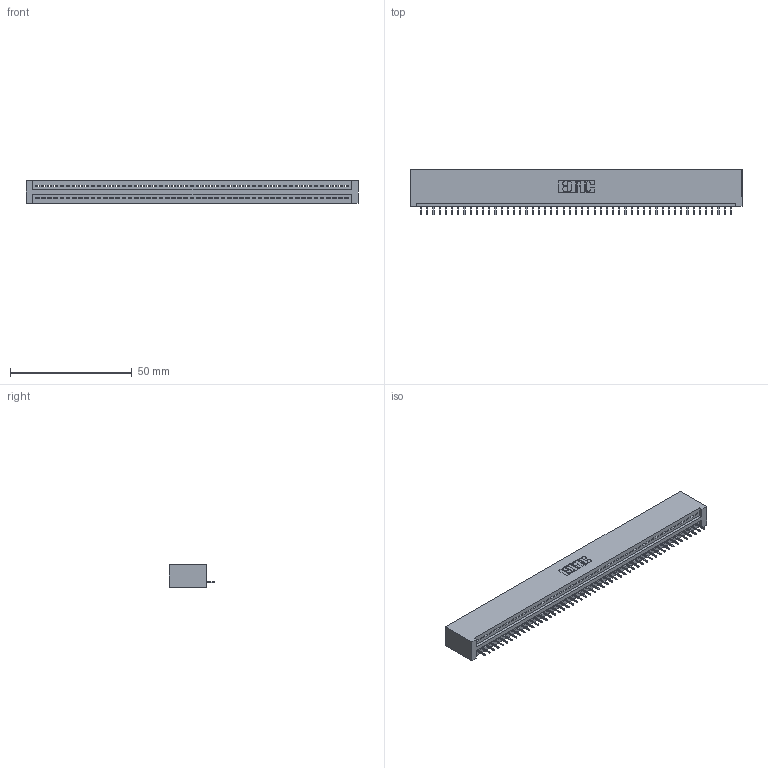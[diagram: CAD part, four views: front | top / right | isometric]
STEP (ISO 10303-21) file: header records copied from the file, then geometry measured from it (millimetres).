
FILE_DESCRIPTION (( 'STEP AP203' ), '1' );
FILE_NAME ('895-051-525-101.STEP', '2020-09-27T10:22:33', ( '' ), ( '' ), 'SwSTEP 2.0', 'SolidWorks 2020', '' );
FILE_SCHEMA (( 'CONFIG_CONTROL_DESIGN' ));
Length unit declared in the file: inch
Products named in the file (3): 345-292-001_345-293-125; 895-051-525-101; 845 Part_No Mounting Lugs
Assembly tree (52 placements, depth 2):
  895-051-525-101
    845 Part_No Mounting Lugs
    345-292-001_345-293-125  x51
Bounding box: 136.14 x 18.72 x 9.4 mm (x, y, z)
Volume: 13381 mm3; surface area: 17400.1 mm2
Topology: 52 solids, 52 shells, 3280 faces, 9497 edges, 6126 vertices
Faces by surface type: plane 2422, cylinder 858
Entity records: 36969 total; most frequent: CARTESIAN_POINT 6409, ORIENTED_EDGE 6394, DIRECTION 5579, EDGE_CURVE 3197, VECTOR 2873, LINE 2873, VERTEX_POINT 2126, AXIS2_PLACEMENT_3D 1353
